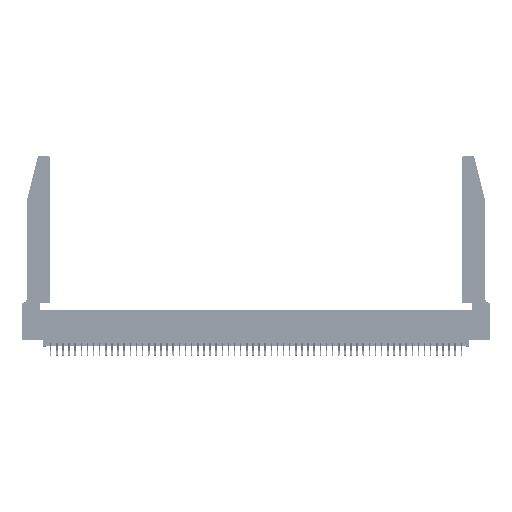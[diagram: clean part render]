
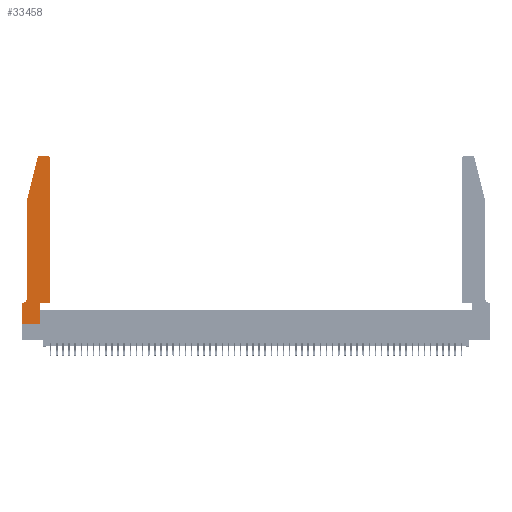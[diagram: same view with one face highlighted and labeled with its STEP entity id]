
A CAD part, top view. The second image highlights one B-rep face of the part: STEP entity #33458.
In plain terms, the highlighted planar face has unit normal (0, 0, 1).
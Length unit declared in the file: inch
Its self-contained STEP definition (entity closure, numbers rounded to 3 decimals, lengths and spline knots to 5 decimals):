
#8 = CARTESIAN_POINT ( 'NONE',  ( 0.0755, 2., 0.37 ) ) ;
#552 = DIRECTION ( 'NONE',  ( 0., 1., 0. ) ) ;
#713 = CARTESIAN_POINT ( 'NONE',  ( 0.2865, 0., 0.37 ) ) ;
#909 = DIRECTION ( 'NONE',  ( -1., 0., 0. ) ) ;
#1023 = VECTOR ( 'NONE', #12269, 39.37008 ) ;
#1182 = ORIENTED_EDGE ( 'NONE', *, *, #46311, .T. ) ;
#2668 = CARTESIAN_POINT ( 'NONE',  ( 0.4505, 0.35, 0.37 ) ) ;
#3686 = VECTOR ( 'NONE', #24046, 39.37008 ) ;
#3702 = CARTESIAN_POINT ( 'NONE',  ( 0.0055, 0.35, 0.37 ) ) ;
#4445 = VERTEX_POINT ( 'NONE', #42542 ) ;
#4578 = CARTESIAN_POINT ( 'NONE',  ( 0.0755, 2., 0.37 ) ) ;
#5602 = LINE ( 'NONE', #54461, #1023 ) ;
#5653 = LINE ( 'NONE', #10841, #3686 ) ;
#6324 = EDGE_CURVE ( 'NONE', #24779, #52675, #35525, .T. ) ;
#8270 = VECTOR ( 'NONE', #552, 39.37008 ) ;
#8788 = CARTESIAN_POINT ( 'NONE',  ( 0., 0., 0.37 ) ) ;
#8984 = DIRECTION ( 'NONE',  ( 0., 1., 0. ) ) ;
#9541 = LINE ( 'NONE', #50450, #53416 ) ;
#9898 = ORIENTED_EDGE ( 'NONE', *, *, #45172, .T. ) ;
#10204 = VECTOR ( 'NONE', #909, 39.37008 ) ;
#10841 = CARTESIAN_POINT ( 'NONE',  ( 0.0755, 2., 0.37 ) ) ;
#11003 = CIRCLE ( 'NONE', #34511, 0.07 ) ;
#11936 = DIRECTION ( 'NONE',  ( 1., 0., 0. ) ) ;
#12213 = EDGE_CURVE ( 'NONE', #46078, #45346, #25804, .T. ) ;
#12269 = DIRECTION ( 'NONE',  ( 0., -1., 0. ) ) ;
#12864 = EDGE_CURVE ( 'NONE', #45346, #38307, #48964, .T. ) ;
#13017 = LINE ( 'NONE', #2668, #34290 ) ;
#15409 = LINE ( 'NONE', #8788, #30668 ) ;
#16240 = ORIENTED_EDGE ( 'NONE', *, *, #28856, .T. ) ;
#16461 = EDGE_CURVE ( 'NONE', #19251, #4445, #45977, .T. ) ;
#16846 = CARTESIAN_POINT ( 'NONE',  ( 0., 0., 0.37 ) ) ;
#17182 = ORIENTED_EDGE ( 'NONE', *, *, #16461, .T. ) ;
#18143 = VERTEX_POINT ( 'NONE', #16846 ) ;
#18852 = CARTESIAN_POINT ( 'NONE',  ( 0.0755, 0.42, 0.37 ) ) ;
#19251 = VERTEX_POINT ( 'NONE', #713 ) ;
#20728 = CARTESIAN_POINT ( 'NONE',  ( 0., 0.35, 0.37 ) ) ;
#22184 = EDGE_CURVE ( 'NONE', #46754, #33452, #9541, .T. ) ;
#22227 = CARTESIAN_POINT ( 'NONE',  ( 0.2605, 2.75, 0.37 ) ) ;
#22800 = CARTESIAN_POINT ( 'NONE',  ( 0.4205, 2.75, 0.37 ) ) ;
#23773 = AXIS2_PLACEMENT_3D ( 'NONE', #49993, #54317, #11936 ) ;
#24046 = DIRECTION ( 'NONE',  ( 0., -1., 0. ) ) ;
#24779 = VERTEX_POINT ( 'NONE', #40148 ) ;
#25318 = AXIS2_PLACEMENT_3D ( 'NONE', #54678, #29742, #29197 ) ;
#25469 = VERTEX_POINT ( 'NONE', #22800 ) ;
#25804 = CIRCLE ( 'NONE', #25318, 0.03 ) ;
#26439 = DIRECTION ( 'NONE',  ( 1., 0., 0. ) ) ;
#26803 = DIRECTION ( 'NONE',  ( 1., 0., 0. ) ) ;
#27361 = VECTOR ( 'NONE', #8984, 39.37008 ) ;
#28007 = EDGE_CURVE ( 'NONE', #52675, #25469, #39618, .T. ) ;
#28565 = DIRECTION ( 'NONE',  ( -1., 0., 0. ) ) ;
#28856 = EDGE_CURVE ( 'NONE', #33452, #18143, #5602, .T. ) ;
#28938 = ORIENTED_EDGE ( 'NONE', *, *, #6324, .T. ) ;
#29197 = DIRECTION ( 'NONE',  ( 1., 0., 0. ) ) ;
#29207 = PLANE ( 'NONE',  #23773 ) ;
#29742 = DIRECTION ( 'NONE',  ( 0., 0., 1. ) ) ;
#29753 = FACE_OUTER_BOUND ( 'NONE', #45306, .T. ) ;
#29825 = CARTESIAN_POINT ( 'NONE',  ( 0.4505, 0.35, 0.37 ) ) ;
#30284 = EDGE_CURVE ( 'NONE', #25469, #46078, #50032, .T. ) ;
#30668 = VECTOR ( 'NONE', #26439, 39.37008 ) ;
#32749 = ORIENTED_EDGE ( 'NONE', *, *, #22184, .T. ) ;
#33036 = VECTOR ( 'NONE', #34829, 39.37008 ) ;
#33452 = VERTEX_POINT ( 'NONE', #20728 ) ;
#33458 = ADVANCED_FACE ( 'NONE', ( #29753 ), #29207, .T. ) ;
#34224 = ORIENTED_EDGE ( 'NONE', *, *, #39020, .T. ) ;
#34290 = VECTOR ( 'NONE', #49741, 39.37008 ) ;
#34511 = AXIS2_PLACEMENT_3D ( 'NONE', #54063, #45156, #41076 ) ;
#34829 = DIRECTION ( 'NONE',  ( -0.239, -0.971, 0. ) ) ;
#34960 = EDGE_CURVE ( 'NONE', #46703, #46754, #11003, .T. ) ;
#35525 = LINE ( 'NONE', #29825, #8270 ) ;
#36943 = ORIENTED_EDGE ( 'NONE', *, *, #12213, .T. ) ;
#38307 = VERTEX_POINT ( 'NONE', #8 ) ;
#38612 = AXIS2_PLACEMENT_3D ( 'NONE', #46882, #44264, #26803 ) ;
#39020 = EDGE_CURVE ( 'NONE', #18143, #19251, #15409, .T. ) ;
#39618 = CIRCLE ( 'NONE', #38612, 0.03 ) ;
#40060 = ORIENTED_EDGE ( 'NONE', *, *, #12864, .T. ) ;
#40148 = CARTESIAN_POINT ( 'NONE',  ( 0.4505, 0.35, 0.37 ) ) ;
#41076 = DIRECTION ( 'NONE',  ( -1., 0., 0. ) ) ;
#42537 = CARTESIAN_POINT ( 'NONE',  ( 0.25487, 2.72718, 0.37 ) ) ;
#42542 = CARTESIAN_POINT ( 'NONE',  ( 0.2865, 0.35, 0.37 ) ) ;
#43175 = CARTESIAN_POINT ( 'NONE',  ( 0.2865, 0.35, 0.37 ) ) ;
#44126 = CARTESIAN_POINT ( 'NONE',  ( 0.284, 2.75, 0.37 ) ) ;
#44264 = DIRECTION ( 'NONE',  ( 0., 0., 1. ) ) ;
#45156 = DIRECTION ( 'NONE',  ( 0., 0., -1. ) ) ;
#45172 = EDGE_CURVE ( 'NONE', #4445, #24779, #13017, .T. ) ;
#45306 = EDGE_LOOP ( 'NONE', ( #50579, #36943, #40060, #1182, #51515, #32749, #16240, #34224, #17182, #9898, #28938, #53848 ) ) ;
#45346 = VERTEX_POINT ( 'NONE', #42537 ) ;
#45977 = LINE ( 'NONE', #43175, #27361 ) ;
#46078 = VERTEX_POINT ( 'NONE', #44126 ) ;
#46311 = EDGE_CURVE ( 'NONE', #38307, #46703, #5653, .T. ) ;
#46703 = VERTEX_POINT ( 'NONE', #18852 ) ;
#46754 = VERTEX_POINT ( 'NONE', #3702 ) ;
#46882 = CARTESIAN_POINT ( 'NONE',  ( 0.4205, 2.72, 0.37 ) ) ;
#47773 = CARTESIAN_POINT ( 'NONE',  ( 0.4505, 2.72, 0.37 ) ) ;
#48964 = LINE ( 'NONE', #4578, #33036 ) ;
#49741 = DIRECTION ( 'NONE',  ( 1., 0., 0. ) ) ;
#49993 = CARTESIAN_POINT ( 'NONE',  ( 0., 0.35, 0.37 ) ) ;
#50032 = LINE ( 'NONE', #22227, #10204 ) ;
#50450 = CARTESIAN_POINT ( 'NONE',  ( 0.0755, 0.35, 0.37 ) ) ;
#50579 = ORIENTED_EDGE ( 'NONE', *, *, #30284, .T. ) ;
#51515 = ORIENTED_EDGE ( 'NONE', *, *, #34960, .T. ) ;
#52675 = VERTEX_POINT ( 'NONE', #47773 ) ;
#53416 = VECTOR ( 'NONE', #28565, 39.37008 ) ;
#53848 = ORIENTED_EDGE ( 'NONE', *, *, #28007, .T. ) ;
#54063 = CARTESIAN_POINT ( 'NONE',  ( 0.0055, 0.42, 0.37 ) ) ;
#54317 = DIRECTION ( 'NONE',  ( 0., 0., 1. ) ) ;
#54461 = CARTESIAN_POINT ( 'NONE',  ( 0., 0., 0.37 ) ) ;
#54678 = CARTESIAN_POINT ( 'NONE',  ( 0.284, 2.72, 0.37 ) ) ;
